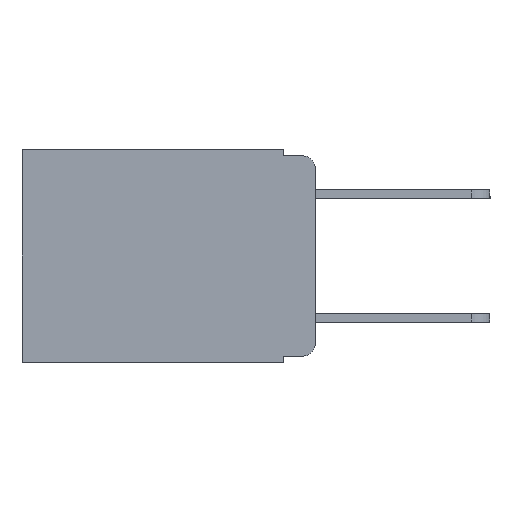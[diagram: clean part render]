
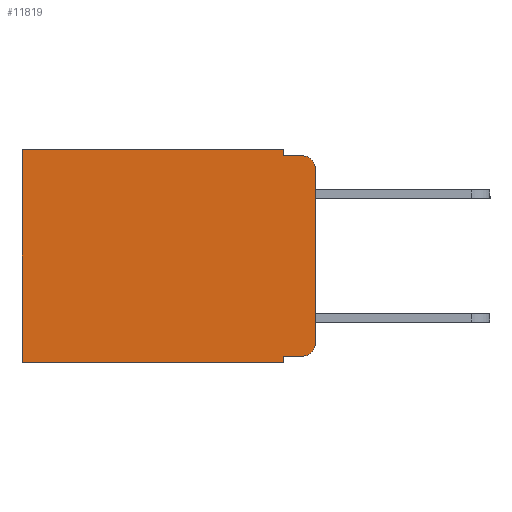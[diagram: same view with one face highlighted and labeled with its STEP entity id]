
A CAD part, left-side view. The second image highlights one B-rep face of the part: STEP entity #11819.
In plain terms, the highlighted planar face has unit normal (-1, 0, 0).
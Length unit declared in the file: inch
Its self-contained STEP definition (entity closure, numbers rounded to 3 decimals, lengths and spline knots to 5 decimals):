
#241 = AXIS2_PLACEMENT_3D ( 'NONE', #1387, #3721, #13420 ) ;
#826 = DIRECTION ( 'NONE',  ( 1., 0., 0. ) ) ;
#1106 = ORIENTED_EDGE ( 'NONE', *, *, #5632, .T. ) ;
#1216 = DIRECTION ( 'NONE',  ( 0., 1., 0. ) ) ;
#1223 = ORIENTED_EDGE ( 'NONE', *, *, #5267, .F. ) ;
#1304 = VERTEX_POINT ( 'NONE', #11241 ) ;
#1387 = CARTESIAN_POINT ( 'NONE',  ( 0.298, 0.02, -0.03 ) ) ;
#1413 = ORIENTED_EDGE ( 'NONE', *, *, #5347, .T. ) ;
#1591 = ORIENTED_EDGE ( 'NONE', *, *, #5340, .F. ) ;
#1624 = LINE ( 'NONE', #10996, #13731 ) ;
#1660 = ORIENTED_EDGE ( 'NONE', *, *, #5351, .T. ) ;
#1948 = DIRECTION ( 'NONE',  ( 0., 1., 0. ) ) ;
#2018 = VERTEX_POINT ( 'NONE', #4518 ) ;
#2537 = LINE ( 'NONE', #2664, #11669 ) ;
#2664 = CARTESIAN_POINT ( 'NONE',  ( 0.298, 0.051, 0. ) ) ;
#2845 = VERTEX_POINT ( 'NONE', #10815 ) ;
#2892 = DIRECTION ( 'NONE',  ( 0., -1., 0. ) ) ;
#2954 = LINE ( 'NONE', #7519, #9000 ) ;
#3721 = DIRECTION ( 'NONE',  ( -1., 0., 0. ) ) ;
#3723 = LINE ( 'NONE', #4102, #9688 ) ;
#3905 = CARTESIAN_POINT ( 'NONE',  ( 0.298, 0.02, -0.313 ) ) ;
#4102 = CARTESIAN_POINT ( 'NONE',  ( 0.298, 0., 0. ) ) ;
#4487 = EDGE_CURVE ( 'NONE', #14900, #1304, #9534, .T. ) ;
#4518 = CARTESIAN_POINT ( 'NONE',  ( 0.298, 0.051, 0. ) ) ;
#4519 = VERTEX_POINT ( 'NONE', #13928 ) ;
#5118 = VECTOR ( 'NONE', #6566, 39.37008 ) ;
#5267 = EDGE_CURVE ( 'NONE', #8104, #8611, #3723, .T. ) ;
#5273 = EDGE_CURVE ( 'NONE', #8104, #11947, #14991, .T. ) ;
#5290 = EDGE_CURVE ( 'NONE', #7478, #11947, #2954, .T. ) ;
#5299 = EDGE_CURVE ( 'NONE', #2018, #7478, #2537, .T. ) ;
#5321 = EDGE_CURVE ( 'NONE', #12565, #1304, #9337, .T. ) ;
#5340 = EDGE_CURVE ( 'NONE', #4519, #14900, #1624, .T. ) ;
#5347 = EDGE_CURVE ( 'NONE', #4519, #2845, #8275, .T. ) ;
#5351 = EDGE_CURVE ( 'NONE', #2845, #8611, #10967, .T. ) ;
#5632 = EDGE_CURVE ( 'NONE', #2018, #12565, #11149, .T. ) ;
#5845 = CARTESIAN_POINT ( 'NONE',  ( 0.298, 0., 0. ) ) ;
#6163 = CARTESIAN_POINT ( 'NONE',  ( 0.298, 0.473, 0. ) ) ;
#6566 = DIRECTION ( 'NONE',  ( 0., -1., 0. ) ) ;
#6842 = VECTOR ( 'NONE', #1948, 39.37008 ) ;
#7478 = VERTEX_POINT ( 'NONE', #12700 ) ;
#7519 = CARTESIAN_POINT ( 'NONE',  ( 0.298, 0.051, -0.01 ) ) ;
#7816 = ORIENTED_EDGE ( 'NONE', *, *, #5321, .T. ) ;
#8104 = VERTEX_POINT ( 'NONE', #10745 ) ;
#8275 = LINE ( 'NONE', #13230, #5118 ) ;
#8373 = FACE_OUTER_BOUND ( 'NONE', #13656, .T. ) ;
#8611 = VERTEX_POINT ( 'NONE', #10970 ) ;
#8625 = VECTOR ( 'NONE', #9560, 39.37008 ) ;
#9000 = VECTOR ( 'NONE', #2892, 39.37008 ) ;
#9337 = LINE ( 'NONE', #6163, #8625 ) ;
#9484 = DIRECTION ( 'NONE',  ( 0., 0., -1. ) ) ;
#9534 = LINE ( 'NONE', #12867, #6842 ) ;
#9560 = DIRECTION ( 'NONE',  ( 0., 0., -1. ) ) ;
#9688 = VECTOR ( 'NONE', #12091, 39.37008 ) ;
#9994 = AXIS2_PLACEMENT_3D ( 'NONE', #10234, #826, #9484 ) ;
#10234 = CARTESIAN_POINT ( 'NONE',  ( 0.298, 0., 0. ) ) ;
#10745 = CARTESIAN_POINT ( 'NONE',  ( 0.298, 0., -0.03 ) ) ;
#10815 = CARTESIAN_POINT ( 'NONE',  ( 0.298, 0.02, -0.333 ) ) ;
#10902 = ORIENTED_EDGE ( 'NONE', *, *, #5299, .F. ) ;
#10905 = DIRECTION ( 'NONE',  ( 0., 0., -1. ) ) ;
#10933 = ORIENTED_EDGE ( 'NONE', *, *, #5273, .T. ) ;
#10967 = CIRCLE ( 'NONE', #14387, 0.02 ) ;
#10970 = CARTESIAN_POINT ( 'NONE',  ( 0.298, 0., -0.313 ) ) ;
#10996 = CARTESIAN_POINT ( 'NONE',  ( 0.298, 0.051, 0. ) ) ;
#11149 = LINE ( 'NONE', #5845, #13563 ) ;
#11241 = CARTESIAN_POINT ( 'NONE',  ( 0.298, 0.473, -0.343 ) ) ;
#11669 = VECTOR ( 'NONE', #15024, 39.37008 ) ;
#11819 = ADVANCED_FACE ( 'NONE', ( #8373 ), #14619, .F. ) ;
#11947 = VERTEX_POINT ( 'NONE', #12366 ) ;
#12091 = DIRECTION ( 'NONE',  ( 0., 0., -1. ) ) ;
#12184 = DIRECTION ( 'NONE',  ( 0., 0., -1. ) ) ;
#12366 = CARTESIAN_POINT ( 'NONE',  ( 0.298, 0.02, -0.01 ) ) ;
#12565 = VERTEX_POINT ( 'NONE', #14597 ) ;
#12700 = CARTESIAN_POINT ( 'NONE',  ( 0.298, 0.051, -0.01 ) ) ;
#12867 = CARTESIAN_POINT ( 'NONE',  ( 0.298, 0., -0.343 ) ) ;
#13064 = CARTESIAN_POINT ( 'NONE',  ( 0.298, 0.051, -0.343 ) ) ;
#13184 = ORIENTED_EDGE ( 'NONE', *, *, #5290, .F. ) ;
#13230 = CARTESIAN_POINT ( 'NONE',  ( 0.298, 0.051, -0.333 ) ) ;
#13420 = DIRECTION ( 'NONE',  ( 0., 0., -1. ) ) ;
#13563 = VECTOR ( 'NONE', #1216, 39.37008 ) ;
#13656 = EDGE_LOOP ( 'NONE', ( #1223, #10933, #13184, #10902, #1106, #7816, #13840, #1591, #1413, #1660 ) ) ;
#13731 = VECTOR ( 'NONE', #12184, 39.37008 ) ;
#13840 = ORIENTED_EDGE ( 'NONE', *, *, #4487, .F. ) ;
#13928 = CARTESIAN_POINT ( 'NONE',  ( 0.298, 0.051, -0.333 ) ) ;
#14081 = DIRECTION ( 'NONE',  ( -1., 0., 0. ) ) ;
#14387 = AXIS2_PLACEMENT_3D ( 'NONE', #3905, #14081, #10905 ) ;
#14597 = CARTESIAN_POINT ( 'NONE',  ( 0.298, 0.473, 0. ) ) ;
#14619 = PLANE ( 'NONE',  #9994 ) ;
#14900 = VERTEX_POINT ( 'NONE', #13064 ) ;
#14991 = CIRCLE ( 'NONE', #241, 0.02 ) ;
#15024 = DIRECTION ( 'NONE',  ( 0., 0., -1. ) ) ;
